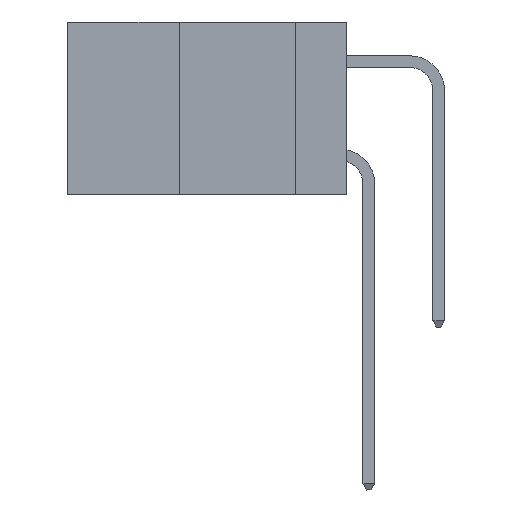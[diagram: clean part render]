
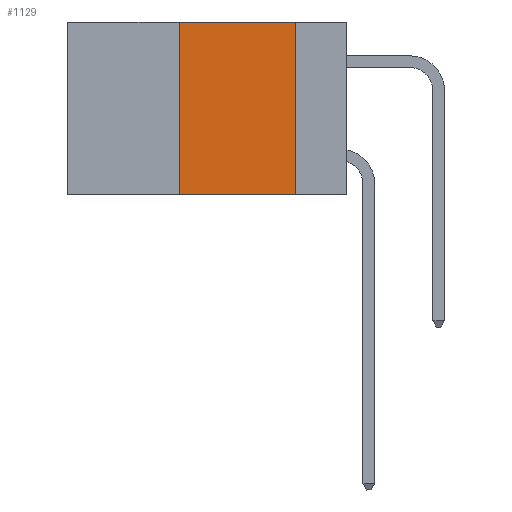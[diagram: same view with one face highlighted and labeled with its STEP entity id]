
A CAD part, left-side view. The second image highlights one B-rep face of the part: STEP entity #1129.
In plain terms, the highlighted planar face has unit normal (-1, 0, 0).
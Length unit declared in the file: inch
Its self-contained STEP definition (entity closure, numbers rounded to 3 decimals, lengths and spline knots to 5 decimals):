
#115 = EDGE_CURVE ( 'NONE', #14078, #6644, #13723, .T. ) ;
#563 = CARTESIAN_POINT ( 'NONE',  ( 0., 0.36, 0. ) ) ;
#1129 = ADVANCED_FACE ( 'NONE', ( #3448 ), #6258, .F. ) ;
#1321 = EDGE_CURVE ( 'NONE', #6644, #14313, #22896, .T. ) ;
#1477 = EDGE_CURVE ( 'NONE', #14313, #15482, #10778, .T. ) ;
#1914 = CARTESIAN_POINT ( 'NONE',  ( 0., 0.36, 0. ) ) ;
#2508 = EDGE_LOOP ( 'NONE', ( #12484, #6738, #3558, #4610 ) ) ;
#3448 = FACE_OUTER_BOUND ( 'NONE', #2508, .T. ) ;
#3558 = ORIENTED_EDGE ( 'NONE', *, *, #115, .F. ) ;
#4032 = DIRECTION ( 'NONE',  ( 0., -1., 0. ) ) ;
#4247 = CARTESIAN_POINT ( 'NONE',  ( 0., 0.11, 0. ) ) ;
#4610 = ORIENTED_EDGE ( 'NONE', *, *, #22892, .T. ) ;
#5385 = CARTESIAN_POINT ( 'NONE',  ( 0., 0.11, -0.37 ) ) ;
#6224 = DIRECTION ( 'NONE',  ( 1., 0., 0. ) ) ;
#6258 = PLANE ( 'NONE',  #14509 ) ;
#6644 = VERTEX_POINT ( 'NONE', #1914 ) ;
#6738 = ORIENTED_EDGE ( 'NONE', *, *, #1321, .F. ) ;
#8220 = CARTESIAN_POINT ( 'NONE',  ( 0., 0.6, -0.37 ) ) ;
#10206 = VECTOR ( 'NONE', #16621, 39.37008 ) ;
#10778 = LINE ( 'NONE', #4247, #10206 ) ;
#10813 = CARTESIAN_POINT ( 'NONE',  ( 0., 0.36, -0.37 ) ) ;
#11780 = DIRECTION ( 'NONE',  ( 0., 0., 1. ) ) ;
#11851 = VECTOR ( 'NONE', #21190, 39.37008 ) ;
#12484 = ORIENTED_EDGE ( 'NONE', *, *, #1477, .F. ) ;
#12576 = DIRECTION ( 'NONE',  ( 0., 0., -1. ) ) ;
#13407 = CARTESIAN_POINT ( 'NONE',  ( 0., 0.6, 0. ) ) ;
#13723 = LINE ( 'NONE', #563, #17525 ) ;
#14078 = VERTEX_POINT ( 'NONE', #10813 ) ;
#14313 = VERTEX_POINT ( 'NONE', #15137 ) ;
#14509 = AXIS2_PLACEMENT_3D ( 'NONE', #13407, #6224, #12576 ) ;
#15137 = CARTESIAN_POINT ( 'NONE',  ( 0., 0.11, 0. ) ) ;
#15482 = VERTEX_POINT ( 'NONE', #5385 ) ;
#16621 = DIRECTION ( 'NONE',  ( 0., 0., -1. ) ) ;
#17525 = VECTOR ( 'NONE', #11780, 39.37008 ) ;
#18018 = VECTOR ( 'NONE', #4032, 39.37008 ) ;
#21147 = LINE ( 'NONE', #8220, #11851 ) ;
#21190 = DIRECTION ( 'NONE',  ( 0., -1., 0. ) ) ;
#22892 = EDGE_CURVE ( 'NONE', #14078, #15482, #21147, .T. ) ;
#22896 = LINE ( 'NONE', #24060, #18018 ) ;
#24060 = CARTESIAN_POINT ( 'NONE',  ( 0., 0.6, 0. ) ) ;
